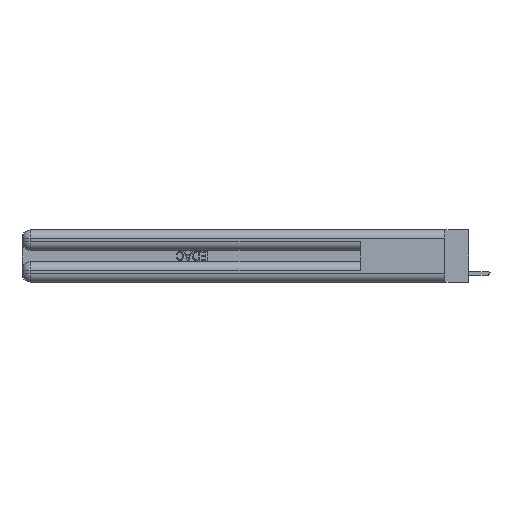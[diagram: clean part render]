
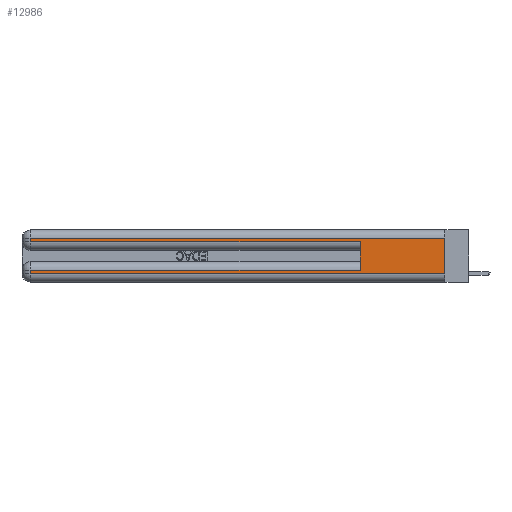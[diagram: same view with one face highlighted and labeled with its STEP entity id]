
A CAD part, left-side view. The second image highlights one B-rep face of the part: STEP entity #12986.
In plain terms, the highlighted planar face has unit normal (-1, 0, 0).
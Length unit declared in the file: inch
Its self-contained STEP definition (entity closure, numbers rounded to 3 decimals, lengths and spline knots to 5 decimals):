
#466 = DIRECTION ( 'NONE',  ( 0., 1., 0. ) ) ;
#1005 = AXIS2_PLACEMENT_3D ( 'NONE', #9587, #25517, #16544 ) ;
#1629 = CARTESIAN_POINT ( 'NONE',  ( 0., 0., 0.06 ) ) ;
#3250 = VECTOR ( 'NONE', #10079, 39.37008 ) ;
#3621 = ORIENTED_EDGE ( 'NONE', *, *, #22174, .F. ) ;
#4048 = LINE ( 'NONE', #16128, #23242 ) ;
#5172 = VERTEX_POINT ( 'NONE', #7747 ) ;
#5559 = CARTESIAN_POINT ( 'NONE',  ( 0., 0.6, 0.285 ) ) ;
#5956 = EDGE_CURVE ( 'NONE', #5172, #27557, #11661, .T. ) ;
#5960 = LINE ( 'NONE', #24333, #11244 ) ;
#6171 = LINE ( 'NONE', #22056, #15403 ) ;
#6204 = CARTESIAN_POINT ( 'NONE',  ( 0., 0.6, 0.145 ) ) ;
#7334 = CARTESIAN_POINT ( 'NONE',  ( 0., 2.94, 0.285 ) ) ;
#7440 = EDGE_CURVE ( 'NONE', #20115, #27557, #13736, .T. ) ;
#7747 = CARTESIAN_POINT ( 'NONE',  ( 0., 0.6, 0.085 ) ) ;
#9131 = VECTOR ( 'NONE', #18107, 39.37008 ) ;
#9587 = CARTESIAN_POINT ( 'NONE',  ( 0., 0., 0.37 ) ) ;
#9841 = CARTESIAN_POINT ( 'NONE',  ( 0., 0., 0.37 ) ) ;
#9985 = CARTESIAN_POINT ( 'NONE',  ( 0., 2.94, 0.37 ) ) ;
#10079 = DIRECTION ( 'NONE',  ( 0., 0., -1. ) ) ;
#10445 = FACE_OUTER_BOUND ( 'NONE', #22974, .T. ) ;
#10746 = CARTESIAN_POINT ( 'NONE',  ( 0., 0., 0.285 ) ) ;
#11221 = VERTEX_POINT ( 'NONE', #1629 ) ;
#11244 = VECTOR ( 'NONE', #27822, 39.37008 ) ;
#11661 = LINE ( 'NONE', #6204, #28108 ) ;
#11694 = DIRECTION ( 'NONE',  ( 0., 0., 1. ) ) ;
#12168 = EDGE_CURVE ( 'NONE', #14970, #20415, #24051, .T. ) ;
#12811 = ORIENTED_EDGE ( 'NONE', *, *, #20154, .T. ) ;
#12986 = ADVANCED_FACE ( 'NONE', ( #10445 ), #18608, .F. ) ;
#13736 = LINE ( 'NONE', #10746, #9131 ) ;
#13905 = EDGE_CURVE ( 'NONE', #20415, #11221, #6171, .T. ) ;
#14630 = LINE ( 'NONE', #9985, #3250 ) ;
#14843 = ORIENTED_EDGE ( 'NONE', *, *, #7440, .T. ) ;
#14970 = VERTEX_POINT ( 'NONE', #24468 ) ;
#15228 = CARTESIAN_POINT ( 'NONE',  ( 0., 2.94, 0.31 ) ) ;
#15309 = DIRECTION ( 'NONE',  ( 0., -1., 0. ) ) ;
#15403 = VECTOR ( 'NONE', #15309, 39.37008 ) ;
#15901 = CARTESIAN_POINT ( 'NONE',  ( 0., 2.94, 0.37 ) ) ;
#16057 = ORIENTED_EDGE ( 'NONE', *, *, #12168, .T. ) ;
#16128 = CARTESIAN_POINT ( 'NONE',  ( 0., 0., 0.085 ) ) ;
#16544 = DIRECTION ( 'NONE',  ( 0., 0., -1. ) ) ;
#17093 = ORIENTED_EDGE ( 'NONE', *, *, #13905, .T. ) ;
#18107 = DIRECTION ( 'NONE',  ( 0., -1., 0. ) ) ;
#18259 = VERTEX_POINT ( 'NONE', #21321 ) ;
#18608 = PLANE ( 'NONE',  #1005 ) ;
#18709 = EDGE_CURVE ( 'NONE', #5172, #14970, #4048, .T. ) ;
#19287 = ORIENTED_EDGE ( 'NONE', *, *, #23766, .T. ) ;
#20115 = VERTEX_POINT ( 'NONE', #7334 ) ;
#20154 = EDGE_CURVE ( 'NONE', #21802, #20115, #14630, .T. ) ;
#20415 = VERTEX_POINT ( 'NONE', #24996 ) ;
#21211 = ORIENTED_EDGE ( 'NONE', *, *, #5956, .F. ) ;
#21321 = CARTESIAN_POINT ( 'NONE',  ( 0., 0., 0.31 ) ) ;
#21802 = VERTEX_POINT ( 'NONE', #15228 ) ;
#21897 = VECTOR ( 'NONE', #22643, 39.37008 ) ;
#22056 = CARTESIAN_POINT ( 'NONE',  ( 0., 0., 0.06 ) ) ;
#22174 = EDGE_CURVE ( 'NONE', #18259, #11221, #28147, .T. ) ;
#22643 = DIRECTION ( 'NONE',  ( 0., 0., -1. ) ) ;
#22974 = EDGE_LOOP ( 'NONE', ( #3621, #19287, #12811, #14843, #21211, #29416, #16057, #17093 ) ) ;
#23242 = VECTOR ( 'NONE', #466, 39.37008 ) ;
#23766 = EDGE_CURVE ( 'NONE', #18259, #21802, #5960, .T. ) ;
#24051 = LINE ( 'NONE', #15901, #21897 ) ;
#24333 = CARTESIAN_POINT ( 'NONE',  ( 0., 0., 0.31 ) ) ;
#24468 = CARTESIAN_POINT ( 'NONE',  ( 0., 2.94, 0.085 ) ) ;
#24996 = CARTESIAN_POINT ( 'NONE',  ( 0., 2.94, 0.06 ) ) ;
#25517 = DIRECTION ( 'NONE',  ( 1., 0., 0. ) ) ;
#26710 = VECTOR ( 'NONE', #27867, 39.37008 ) ;
#27557 = VERTEX_POINT ( 'NONE', #5559 ) ;
#27822 = DIRECTION ( 'NONE',  ( 0., 1., 0. ) ) ;
#27867 = DIRECTION ( 'NONE',  ( 0., 0., -1. ) ) ;
#28108 = VECTOR ( 'NONE', #11694, 39.37008 ) ;
#28147 = LINE ( 'NONE', #9841, #26710 ) ;
#29416 = ORIENTED_EDGE ( 'NONE', *, *, #18709, .T. ) ;
